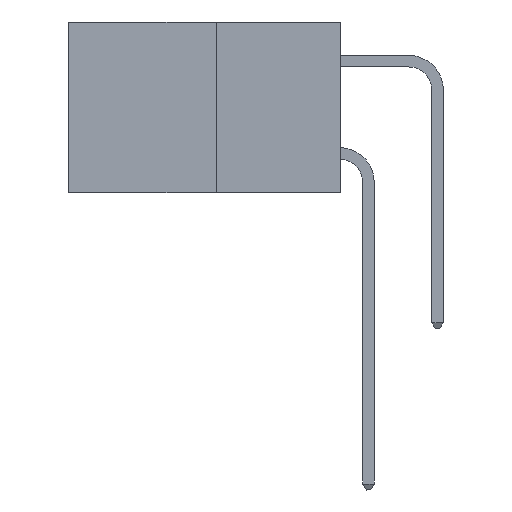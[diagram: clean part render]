
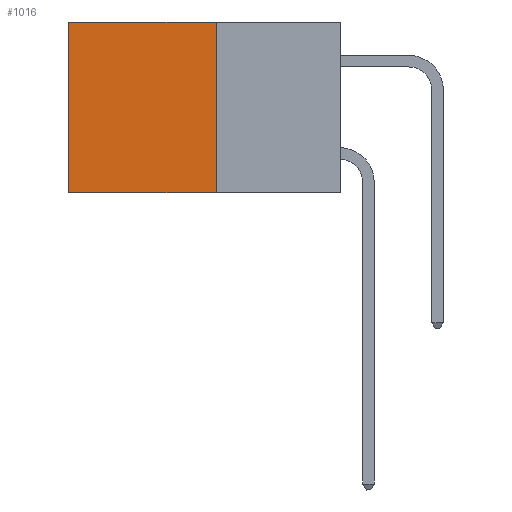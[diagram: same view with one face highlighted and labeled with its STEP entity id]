
A CAD part, left-side view. The second image highlights one B-rep face of the part: STEP entity #1016.
In plain terms, the highlighted planar face has unit normal (-1, 0, 0).
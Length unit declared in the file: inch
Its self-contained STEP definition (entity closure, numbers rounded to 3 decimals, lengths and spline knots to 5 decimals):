
#410 = CARTESIAN_POINT ( 'NONE',  ( 0.277, 0.27, -0.37 ) ) ;
#898 = LINE ( 'NONE', #24044, #6390 ) ;
#1016 = ADVANCED_FACE ( 'NONE', ( #17182 ), #21028, .F. ) ;
#1830 = CARTESIAN_POINT ( 'NONE',  ( 0.277, 0.27, -0.37 ) ) ;
#1867 = DIRECTION ( 'NONE',  ( 1., 0., 0. ) ) ;
#1873 = DIRECTION ( 'NONE',  ( 0., 0., -1. ) ) ;
#2252 = ORIENTED_EDGE ( 'NONE', *, *, #27919, .T. ) ;
#2673 = CARTESIAN_POINT ( 'NONE',  ( 0.277, 0.27, 0. ) ) ;
#4563 = EDGE_CURVE ( 'NONE', #10751, #17709, #898, .T. ) ;
#6124 = CARTESIAN_POINT ( 'NONE',  ( 0.277, 0.27, 0. ) ) ;
#6390 = VECTOR ( 'NONE', #16971, 39.37008 ) ;
#6882 = EDGE_CURVE ( 'NONE', #28844, #17709, #23953, .T. ) ;
#8269 = VERTEX_POINT ( 'NONE', #2673 ) ;
#8289 = EDGE_LOOP ( 'NONE', ( #11360, #25294, #30037, #2252 ) ) ;
#8505 = DIRECTION ( 'NONE',  ( 0., 1., 0. ) ) ;
#9572 = VECTOR ( 'NONE', #8505, 39.37008 ) ;
#10751 = VERTEX_POINT ( 'NONE', #11465 ) ;
#11360 = ORIENTED_EDGE ( 'NONE', *, *, #4563, .T. ) ;
#11465 = CARTESIAN_POINT ( 'NONE',  ( 0.277, 0.59, 0. ) ) ;
#11763 = LINE ( 'NONE', #6124, #9572 ) ;
#16856 = DIRECTION ( 'NONE',  ( 0., 1., 0. ) ) ;
#16971 = DIRECTION ( 'NONE',  ( 0., 0., -1. ) ) ;
#17182 = FACE_OUTER_BOUND ( 'NONE', #8289, .T. ) ;
#17400 = AXIS2_PLACEMENT_3D ( 'NONE', #1830, #1867, #1873 ) ;
#17709 = VERTEX_POINT ( 'NONE', #22420 ) ;
#21028 = PLANE ( 'NONE',  #17400 ) ;
#22409 = DIRECTION ( 'NONE',  ( 0., 0., -1. ) ) ;
#22420 = CARTESIAN_POINT ( 'NONE',  ( 0.277, 0.59, -0.37 ) ) ;
#23227 = VECTOR ( 'NONE', #16856, 39.37008 ) ;
#23953 = LINE ( 'NONE', #410, #23227 ) ;
#24044 = CARTESIAN_POINT ( 'NONE',  ( 0.277, 0.59, -0.37 ) ) ;
#25294 = ORIENTED_EDGE ( 'NONE', *, *, #6882, .F. ) ;
#25759 = CARTESIAN_POINT ( 'NONE',  ( 0.277, 0.27, -0.37 ) ) ;
#26428 = VECTOR ( 'NONE', #22409, 39.37008 ) ;
#27146 = LINE ( 'NONE', #29264, #26428 ) ;
#27297 = EDGE_CURVE ( 'NONE', #8269, #28844, #27146, .T. ) ;
#27919 = EDGE_CURVE ( 'NONE', #8269, #10751, #11763, .T. ) ;
#28844 = VERTEX_POINT ( 'NONE', #25759 ) ;
#29264 = CARTESIAN_POINT ( 'NONE',  ( 0.277, 0.27, -0.37 ) ) ;
#30037 = ORIENTED_EDGE ( 'NONE', *, *, #27297, .F. ) ;
